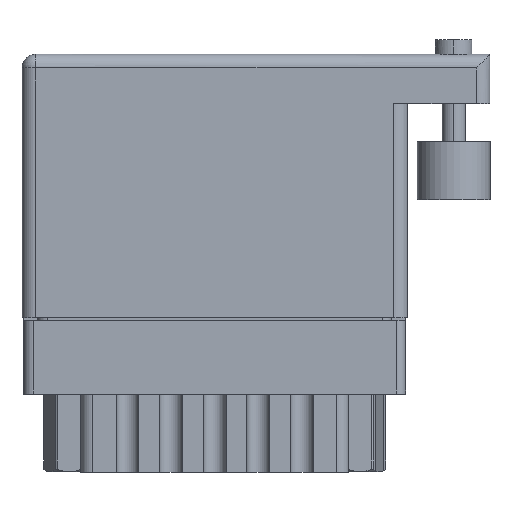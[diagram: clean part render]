
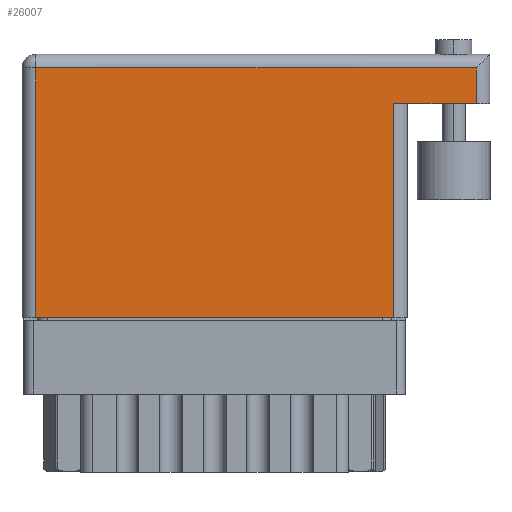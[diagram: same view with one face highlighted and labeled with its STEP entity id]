
A CAD part, front view. The second image highlights one B-rep face of the part: STEP entity #26007.
In plain terms, the highlighted face is planar.
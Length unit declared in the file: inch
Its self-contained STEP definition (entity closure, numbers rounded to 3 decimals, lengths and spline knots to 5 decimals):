
#181 = ORIENTED_EDGE ( 'NONE', *, *, #9004, .F. ) ;
#1178 = VERTEX_POINT ( 'NONE', #37625 ) ;
#2171 = ORIENTED_EDGE ( 'NONE', *, *, #19430, .T. ) ;
#2861 = DIRECTION ( 'NONE',  ( -1., 0., 0. ) ) ;
#6864 = EDGE_CURVE ( 'NONE', #15985, #23077, #23955, .T. ) ;
#8763 = ORIENTED_EDGE ( 'NONE', *, *, #14057, .T. ) ;
#9004 = EDGE_CURVE ( 'NONE', #27115, #23077, #31852, .T. ) ;
#9331 = CARTESIAN_POINT ( 'NONE',  ( 0.047, 0.859, 0. ) ) ;
#11159 = VECTOR ( 'NONE', #24617, 39.37008 ) ;
#11229 = DIRECTION ( 'NONE',  ( 0., 1., 0. ) ) ;
#12781 = ORIENTED_EDGE ( 'NONE', *, *, #6864, .T. ) ;
#13401 = DIRECTION ( 'NONE',  ( -1., 0., 0. ) ) ;
#13885 = AXIS2_PLACEMENT_3D ( 'NONE', #24889, #37030, #2861 ) ;
#14057 = EDGE_CURVE ( 'NONE', #26883, #32986, #21637, .T. ) ;
#14786 = LINE ( 'NONE', #39021, #15685 ) ;
#15685 = VECTOR ( 'NONE', #11229, 39.37008 ) ;
#15985 = VERTEX_POINT ( 'NONE', #26048 ) ;
#16376 = CARTESIAN_POINT ( 'NONE',  ( 1.609, 0.736, 0. ) ) ;
#16936 = EDGE_CURVE ( 'NONE', #27115, #1178, #14786, .T. ) ;
#18021 = EDGE_LOOP ( 'NONE', ( #20483, #12781, #181, #24633, #2171, #8763 ) ) ;
#18561 = PLANE ( 'NONE',  #13885 ) ;
#18585 = CARTESIAN_POINT ( 'NONE',  ( 1.278, 0.736, 0. ) ) ;
#19430 = EDGE_CURVE ( 'NONE', #1178, #26883, #20769, .T. ) ;
#19861 = LINE ( 'NONE', #29388, #26566 ) ;
#20483 = ORIENTED_EDGE ( 'NONE', *, *, #25720, .T. ) ;
#20769 = LINE ( 'NONE', #27528, #33961 ) ;
#21328 = FACE_OUTER_BOUND ( 'NONE', #18021, .T. ) ;
#21637 = LINE ( 'NONE', #33779, #11159 ) ;
#23077 = VERTEX_POINT ( 'NONE', #18585 ) ;
#23715 = VECTOR ( 'NONE', #33114, 39.37008 ) ;
#23955 = LINE ( 'NONE', #36097, #23715 ) ;
#24617 = DIRECTION ( 'NONE',  ( 0., -1., 0. ) ) ;
#24633 = ORIENTED_EDGE ( 'NONE', *, *, #16936, .T. ) ;
#24889 = CARTESIAN_POINT ( 'NONE',  ( 0., 0.906, 0. ) ) ;
#25720 = EDGE_CURVE ( 'NONE', #32986, #15985, #19861, .T. ) ;
#26007 = ADVANCED_FACE ( 'NONE', ( #21328 ), #18561, .F. ) ;
#26048 = CARTESIAN_POINT ( 'NONE',  ( 1.278, 0., 0. ) ) ;
#26566 = VECTOR ( 'NONE', #31971, 39.37008 ) ;
#26883 = VERTEX_POINT ( 'NONE', #9331 ) ;
#26922 = CARTESIAN_POINT ( 'NONE',  ( 1.562, 0.736, 0. ) ) ;
#27115 = VERTEX_POINT ( 'NONE', #26922 ) ;
#27528 = CARTESIAN_POINT ( 'NONE',  ( 0., 0.859, 0. ) ) ;
#29388 = CARTESIAN_POINT ( 'NONE',  ( 0., 0., 0. ) ) ;
#31852 = LINE ( 'NONE', #16376, #32450 ) ;
#31971 = DIRECTION ( 'NONE',  ( 1., 0., 0. ) ) ;
#32450 = VECTOR ( 'NONE', #13401, 39.37008 ) ;
#32700 = DIRECTION ( 'NONE',  ( -1., 0., 0. ) ) ;
#32986 = VERTEX_POINT ( 'NONE', #34377 ) ;
#33114 = DIRECTION ( 'NONE',  ( 0., 1., 0. ) ) ;
#33779 = CARTESIAN_POINT ( 'NONE',  ( 0.047, 0., 0. ) ) ;
#33961 = VECTOR ( 'NONE', #32700, 39.37008 ) ;
#34377 = CARTESIAN_POINT ( 'NONE',  ( 0.047, 0., 0. ) ) ;
#36097 = CARTESIAN_POINT ( 'NONE',  ( 1.278, 0.736, 0. ) ) ;
#37030 = DIRECTION ( 'NONE',  ( 0., 0., -1. ) ) ;
#37625 = CARTESIAN_POINT ( 'NONE',  ( 1.562, 0.859, 0. ) ) ;
#39021 = CARTESIAN_POINT ( 'NONE',  ( 1.562, 0.906, 0. ) ) ;
